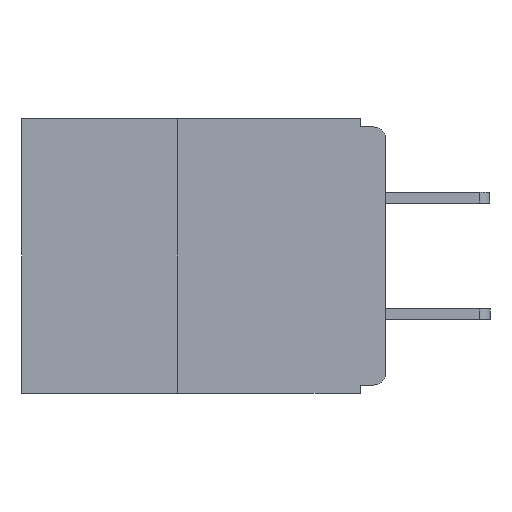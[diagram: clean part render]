
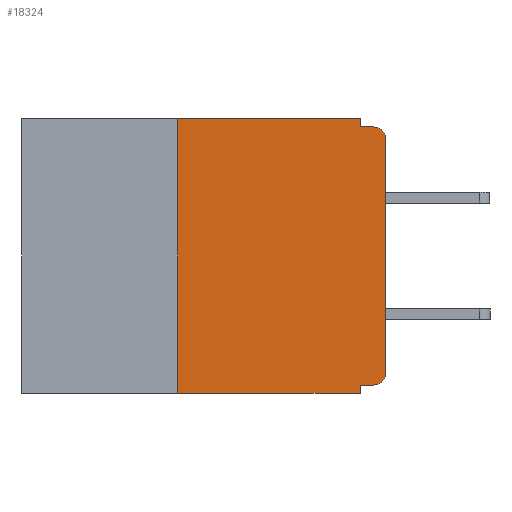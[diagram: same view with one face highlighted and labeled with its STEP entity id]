
A CAD part, left-side view. The second image highlights one B-rep face of the part: STEP entity #18324.
In plain terms, the highlighted planar face has unit normal (-1, 0, 0).
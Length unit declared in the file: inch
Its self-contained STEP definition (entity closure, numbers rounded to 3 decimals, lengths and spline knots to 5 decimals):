
#169 = CARTESIAN_POINT ( 'NONE',  ( 0., 0.25, -0.33 ) ) ;
#244 = LINE ( 'NONE', #28268, #7675 ) ;
#949 = VECTOR ( 'NONE', #25566, 39.37008 ) ;
#1110 = ORIENTED_EDGE ( 'NONE', *, *, #24024, .T. ) ;
#1556 = VECTOR ( 'NONE', #23655, 39.37008 ) ;
#2904 = VERTEX_POINT ( 'NONE', #26028 ) ;
#3903 = AXIS2_PLACEMENT_3D ( 'NONE', #31248, #15413, #33767 ) ;
#5064 = ORIENTED_EDGE ( 'NONE', *, *, #5456, .F. ) ;
#5129 = ORIENTED_EDGE ( 'NONE', *, *, #21889, .F. ) ;
#5353 = ORIENTED_EDGE ( 'NONE', *, *, #5714, .F. ) ;
#5396 = VERTEX_POINT ( 'NONE', #26756 ) ;
#5456 = EDGE_CURVE ( 'NONE', #21622, #13012, #8006, .T. ) ;
#5562 = CARTESIAN_POINT ( 'NONE',  ( 0., 0.437, -0.33 ) ) ;
#5714 = EDGE_CURVE ( 'NONE', #17180, #2904, #33301, .T. ) ;
#5771 = ORIENTED_EDGE ( 'NONE', *, *, #21944, .F. ) ;
#5933 = AXIS2_PLACEMENT_3D ( 'NONE', #24937, #30264, #14387 ) ;
#6149 = EDGE_CURVE ( 'NONE', #26666, #26139, #22704, .T. ) ;
#6570 = EDGE_CURVE ( 'NONE', #5396, #14345, #29691, .T. ) ;
#7581 = CIRCLE ( 'NONE', #32631, 0.015 ) ;
#7675 = VECTOR ( 'NONE', #12221, 39.37008 ) ;
#8006 = LINE ( 'NONE', #13639, #13545 ) ;
#8197 = ORIENTED_EDGE ( 'NONE', *, *, #6149, .T. ) ;
#8276 = DIRECTION ( 'NONE',  ( 0., -1., 0. ) ) ;
#8953 = ORIENTED_EDGE ( 'NONE', *, *, #6570, .F. ) ;
#9881 = CARTESIAN_POINT ( 'NONE',  ( 0., 0., -0.32 ) ) ;
#11654 = PLANE ( 'NONE',  #5933 ) ;
#11705 = CARTESIAN_POINT ( 'NONE',  ( 0., 0.031, -0.33 ) ) ;
#11980 = CARTESIAN_POINT ( 'NONE',  ( 0., 0., -0.025 ) ) ;
#12071 = CARTESIAN_POINT ( 'NONE',  ( 0., 0., -0.01 ) ) ;
#12221 = DIRECTION ( 'NONE',  ( 0., 0., -1. ) ) ;
#12308 = CARTESIAN_POINT ( 'NONE',  ( 0., 0., 0. ) ) ;
#13012 = VERTEX_POINT ( 'NONE', #29785 ) ;
#13545 = VECTOR ( 'NONE', #8276, 39.37008 ) ;
#13639 = CARTESIAN_POINT ( 'NONE',  ( 0., 0.437, 0. ) ) ;
#14343 = EDGE_LOOP ( 'NONE', ( #1110, #16128, #5353, #5129, #5064, #5771, #8197, #16244, #8953, #31050 ) ) ;
#14345 = VERTEX_POINT ( 'NONE', #22006 ) ;
#14387 = DIRECTION ( 'NONE',  ( 0., 0., -1. ) ) ;
#14736 = VECTOR ( 'NONE', #15214, 39.37008 ) ;
#14803 = DIRECTION ( 'NONE',  ( 0., -1., 0. ) ) ;
#15157 = CARTESIAN_POINT ( 'NONE',  ( 0., 0.25, -0.33 ) ) ;
#15214 = DIRECTION ( 'NONE',  ( 0., 1., 0. ) ) ;
#15284 = CARTESIAN_POINT ( 'NONE',  ( 0., 0., -0.305 ) ) ;
#15413 = DIRECTION ( 'NONE',  ( -1., 0., 0. ) ) ;
#15928 = FACE_OUTER_BOUND ( 'NONE', #14343, .T. ) ;
#16128 = ORIENTED_EDGE ( 'NONE', *, *, #30211, .T. ) ;
#16244 = ORIENTED_EDGE ( 'NONE', *, *, #22049, .F. ) ;
#16367 = DIRECTION ( 'NONE',  ( -1., 0., 0. ) ) ;
#17180 = VERTEX_POINT ( 'NONE', #33331 ) ;
#17248 = LINE ( 'NONE', #12308, #949 ) ;
#17855 = DIRECTION ( 'NONE',  ( 0., 0., 1. ) ) ;
#18324 = ADVANCED_FACE ( 'NONE', ( #15928 ), #11654, .F. ) ;
#21030 = VECTOR ( 'NONE', #24399, 39.37008 ) ;
#21622 = VERTEX_POINT ( 'NONE', #29704 ) ;
#21889 = EDGE_CURVE ( 'NONE', #13012, #17180, #244, .T. ) ;
#21944 = EDGE_CURVE ( 'NONE', #26666, #21622, #27349, .T. ) ;
#21978 = VERTEX_POINT ( 'NONE', #15284 ) ;
#22006 = CARTESIAN_POINT ( 'NONE',  ( 0., 0.031, -0.32 ) ) ;
#22049 = EDGE_CURVE ( 'NONE', #14345, #26139, #23233, .T. ) ;
#22704 = LINE ( 'NONE', #5562, #21030 ) ;
#23233 = LINE ( 'NONE', #28850, #1556 ) ;
#23257 = EDGE_CURVE ( 'NONE', #5396, #21978, #7581, .T. ) ;
#23485 = VERTEX_POINT ( 'NONE', #11980 ) ;
#23655 = DIRECTION ( 'NONE',  ( 0., 0., -1. ) ) ;
#24024 = EDGE_CURVE ( 'NONE', #21978, #23485, #17248, .T. ) ;
#24399 = DIRECTION ( 'NONE',  ( 0., -1., 0. ) ) ;
#24937 = CARTESIAN_POINT ( 'NONE',  ( 0., 0.437, 0. ) ) ;
#25566 = DIRECTION ( 'NONE',  ( 0., 0., 1. ) ) ;
#26028 = CARTESIAN_POINT ( 'NONE',  ( 0., 0.015, -0.01 ) ) ;
#26139 = VERTEX_POINT ( 'NONE', #11705 ) ;
#26416 = VECTOR ( 'NONE', #14803, 39.37008 ) ;
#26525 = VECTOR ( 'NONE', #17855, 39.37008 ) ;
#26666 = VERTEX_POINT ( 'NONE', #169 ) ;
#26756 = CARTESIAN_POINT ( 'NONE',  ( 0., 0.015, -0.32 ) ) ;
#27349 = LINE ( 'NONE', #15157, #26525 ) ;
#28268 = CARTESIAN_POINT ( 'NONE',  ( 0., 0.031, 0. ) ) ;
#28850 = CARTESIAN_POINT ( 'NONE',  ( 0., 0.031, -0.33 ) ) ;
#29691 = LINE ( 'NONE', #9881, #14736 ) ;
#29704 = CARTESIAN_POINT ( 'NONE',  ( 0., 0.25, 0. ) ) ;
#29785 = CARTESIAN_POINT ( 'NONE',  ( 0., 0.031, 0. ) ) ;
#30211 = EDGE_CURVE ( 'NONE', #23485, #2904, #33429, .T. ) ;
#30264 = DIRECTION ( 'NONE',  ( 1., 0., 0. ) ) ;
#31050 = ORIENTED_EDGE ( 'NONE', *, *, #23257, .T. ) ;
#31248 = CARTESIAN_POINT ( 'NONE',  ( 0., 0.015, -0.025 ) ) ;
#32131 = CARTESIAN_POINT ( 'NONE',  ( 0., 0.015, -0.305 ) ) ;
#32631 = AXIS2_PLACEMENT_3D ( 'NONE', #32131, #16367, #34641 ) ;
#33301 = LINE ( 'NONE', #12071, #26416 ) ;
#33331 = CARTESIAN_POINT ( 'NONE',  ( 0., 0.031, -0.01 ) ) ;
#33429 = CIRCLE ( 'NONE', #3903, 0.015 ) ;
#33767 = DIRECTION ( 'NONE',  ( 0., 0., -1. ) ) ;
#34641 = DIRECTION ( 'NONE',  ( 0., 0., -1. ) ) ;
